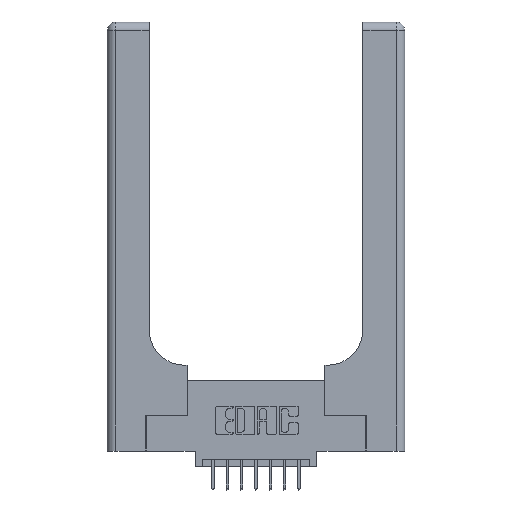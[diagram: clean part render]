
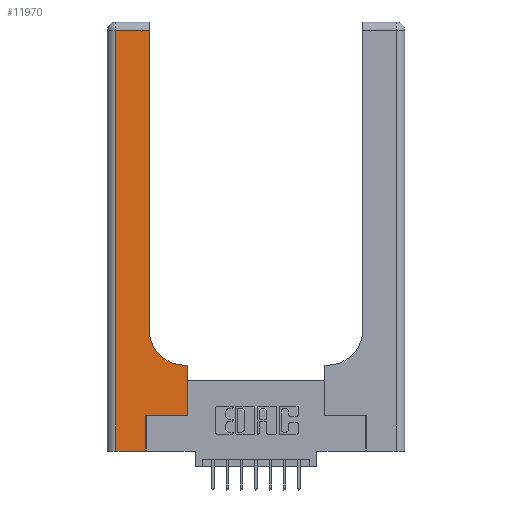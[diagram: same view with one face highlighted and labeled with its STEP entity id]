
A CAD part, top view. The second image highlights one B-rep face of the part: STEP entity #11970.
In plain terms, the highlighted planar face has unit normal (0, 0, 1).
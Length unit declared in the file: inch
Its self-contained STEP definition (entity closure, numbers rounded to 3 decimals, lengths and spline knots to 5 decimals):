
#115 = EDGE_CURVE ( 'NONE', #502, #11172, #11065, .T. ) ;
#219 = VECTOR ( 'NONE', #1738, 39.37008 ) ;
#256 = DIRECTION ( 'NONE',  ( 1., 0., 0. ) ) ;
#342 = EDGE_CURVE ( 'NONE', #13091, #14467, #10296, .T. ) ;
#502 = VERTEX_POINT ( 'NONE', #12164 ) ;
#658 = PLANE ( 'NONE',  #1451 ) ;
#958 = CARTESIAN_POINT ( 'NONE',  ( 0.269, 0.25, 0.37 ) ) ;
#967 = LINE ( 'NONE', #9873, #219 ) ;
#1300 = CARTESIAN_POINT ( 'NONE',  ( 0.5415, 0.85, 0.37 ) ) ;
#1412 = DIRECTION ( 'NONE',  ( 0., 1., 0. ) ) ;
#1451 = AXIS2_PLACEMENT_3D ( 'NONE', #5458, #1880, #10323 ) ;
#1686 = EDGE_LOOP ( 'NONE', ( #10427, #6079, #12406, #3011, #12718, #12758, #13622, #14029, #5431 ) ) ;
#1738 = DIRECTION ( 'NONE',  ( 0., 1., 0. ) ) ;
#1880 = DIRECTION ( 'NONE',  ( 0., 0., -1. ) ) ;
#2843 = EDGE_CURVE ( 'NONE', #11172, #7131, #967, .T. ) ;
#3011 = ORIENTED_EDGE ( 'NONE', *, *, #14030, .T. ) ;
#3114 = EDGE_CURVE ( 'NONE', #15093, #13091, #12668, .T. ) ;
#3280 = EDGE_CURVE ( 'NONE', #7131, #4539, #15472, .T. ) ;
#3320 = CARTESIAN_POINT ( 'NONE',  ( 0.269, 0., 0.37 ) ) ;
#3611 = VERTEX_POINT ( 'NONE', #6843 ) ;
#3825 = CARTESIAN_POINT ( 'NONE',  ( 0.5585, 0.25, 0.37 ) ) ;
#4046 = LINE ( 'NONE', #4253, #10286 ) ;
#4161 = VECTOR ( 'NONE', #6071, 39.37008 ) ;
#4253 = CARTESIAN_POINT ( 'NONE',  ( 0.06, 3., 0.37 ) ) ;
#4539 = VERTEX_POINT ( 'NONE', #12725 ) ;
#4902 = CARTESIAN_POINT ( 'NONE',  ( 0.2915, 0.85, 0.37 ) ) ;
#5228 = CARTESIAN_POINT ( 'NONE',  ( 0.06, 0., 0.37 ) ) ;
#5236 = VECTOR ( 'NONE', #7840, 39.37008 ) ;
#5367 = VECTOR ( 'NONE', #11852, 39.37008 ) ;
#5431 = ORIENTED_EDGE ( 'NONE', *, *, #115, .T. ) ;
#5458 = CARTESIAN_POINT ( 'NONE',  ( 0., 3., 0.37 ) ) ;
#5579 = DIRECTION ( 'NONE',  ( 0., -1., 0. ) ) ;
#5623 = LINE ( 'NONE', #8809, #5236 ) ;
#6071 = DIRECTION ( 'NONE',  ( -1., 0., 0. ) ) ;
#6079 = ORIENTED_EDGE ( 'NONE', *, *, #3280, .T. ) ;
#6491 = VERTEX_POINT ( 'NONE', #5228 ) ;
#6499 = CARTESIAN_POINT ( 'NONE',  ( 0.5585, 0.25, 0.37 ) ) ;
#6843 = CARTESIAN_POINT ( 'NONE',  ( 0.5585, 0.6, 0.37 ) ) ;
#7131 = VERTEX_POINT ( 'NONE', #7140 ) ;
#7140 = CARTESIAN_POINT ( 'NONE',  ( 0.2915, 2.94, 0.37 ) ) ;
#7840 = DIRECTION ( 'NONE',  ( -1., 0., 0. ) ) ;
#8809 = CARTESIAN_POINT ( 'NONE',  ( 0.2915, 0.6, 0.37 ) ) ;
#9357 = AXIS2_PLACEMENT_3D ( 'NONE', #1300, #9757, #14626 ) ;
#9403 = VECTOR ( 'NONE', #256, 39.37008 ) ;
#9757 = DIRECTION ( 'NONE',  ( 0., 0., -1. ) ) ;
#9760 = EDGE_CURVE ( 'NONE', #4539, #6491, #4046, .T. ) ;
#9839 = VECTOR ( 'NONE', #15531, 39.37008 ) ;
#9873 = CARTESIAN_POINT ( 'NONE',  ( 0.2915, 3., 0.37 ) ) ;
#10286 = VECTOR ( 'NONE', #5579, 39.37008 ) ;
#10296 = LINE ( 'NONE', #11802, #5367 ) ;
#10323 = DIRECTION ( 'NONE',  ( -1., 0., 0. ) ) ;
#10427 = ORIENTED_EDGE ( 'NONE', *, *, #2843, .T. ) ;
#10802 = CARTESIAN_POINT ( 'NONE',  ( 0.269, 0., 0.37 ) ) ;
#11065 = CIRCLE ( 'NONE', #9357, 0.25 ) ;
#11164 = EDGE_CURVE ( 'NONE', #14467, #3611, #12689, .T. ) ;
#11172 = VERTEX_POINT ( 'NONE', #4902 ) ;
#11304 = CARTESIAN_POINT ( 'NONE',  ( 0., 0., 0.37 ) ) ;
#11669 = LINE ( 'NONE', #11304, #9403 ) ;
#11802 = CARTESIAN_POINT ( 'NONE',  ( 0.269, 0.25, 0.37 ) ) ;
#11852 = DIRECTION ( 'NONE',  ( 1., 0., 0. ) ) ;
#11970 = ADVANCED_FACE ( 'NONE', ( #13057 ), #658, .F. ) ;
#12164 = CARTESIAN_POINT ( 'NONE',  ( 0.5415, 0.6, 0.37 ) ) ;
#12406 = ORIENTED_EDGE ( 'NONE', *, *, #9760, .T. ) ;
#12668 = LINE ( 'NONE', #3320, #9839 ) ;
#12689 = LINE ( 'NONE', #6499, #14171 ) ;
#12718 = ORIENTED_EDGE ( 'NONE', *, *, #3114, .T. ) ;
#12725 = CARTESIAN_POINT ( 'NONE',  ( 0.06, 2.94, 0.37 ) ) ;
#12758 = ORIENTED_EDGE ( 'NONE', *, *, #342, .T. ) ;
#13057 = FACE_OUTER_BOUND ( 'NONE', #1686, .T. ) ;
#13091 = VERTEX_POINT ( 'NONE', #958 ) ;
#13329 = CARTESIAN_POINT ( 'NONE',  ( 0., 2.94, 0.37 ) ) ;
#13622 = ORIENTED_EDGE ( 'NONE', *, *, #11164, .T. ) ;
#14029 = ORIENTED_EDGE ( 'NONE', *, *, #14692, .T. ) ;
#14030 = EDGE_CURVE ( 'NONE', #6491, #15093, #11669, .T. ) ;
#14171 = VECTOR ( 'NONE', #1412, 39.37008 ) ;
#14467 = VERTEX_POINT ( 'NONE', #3825 ) ;
#14626 = DIRECTION ( 'NONE',  ( 1., 0., 0. ) ) ;
#14692 = EDGE_CURVE ( 'NONE', #3611, #502, #5623, .T. ) ;
#15093 = VERTEX_POINT ( 'NONE', #10802 ) ;
#15472 = LINE ( 'NONE', #13329, #4161 ) ;
#15531 = DIRECTION ( 'NONE',  ( 0., 1., 0. ) ) ;
